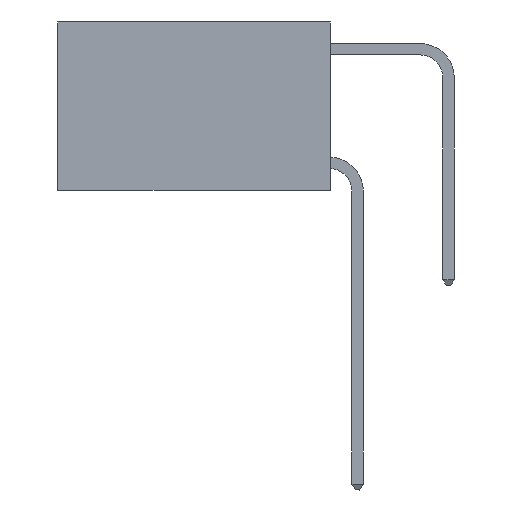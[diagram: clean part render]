
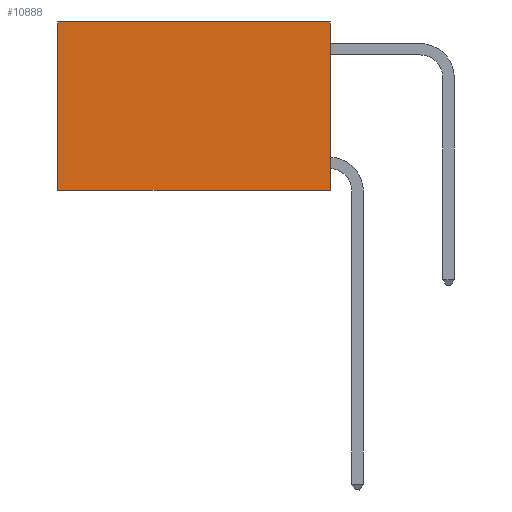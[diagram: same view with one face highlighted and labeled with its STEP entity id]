
A CAD part, left-side view. The second image highlights one B-rep face of the part: STEP entity #10888.
In plain terms, the highlighted planar face has unit normal (-1, 0, 0).
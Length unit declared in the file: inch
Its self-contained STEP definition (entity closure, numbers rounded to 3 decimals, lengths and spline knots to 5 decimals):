
#425 = DIRECTION ( 'NONE',  ( 0., 1., 0. ) ) ;
#703 = DIRECTION ( 'NONE',  ( 0., 0., -1. ) ) ;
#2368 = VECTOR ( 'NONE', #703, 39.37008 ) ;
#4046 = VERTEX_POINT ( 'NONE', #17541 ) ;
#6026 = DIRECTION ( 'NONE',  ( 1., 0., 0. ) ) ;
#7569 = VERTEX_POINT ( 'NONE', #16554 ) ;
#7814 = CARTESIAN_POINT ( 'NONE',  ( 0.2625, 0., -0.37 ) ) ;
#8562 = ORIENTED_EDGE ( 'NONE', *, *, #29483, .T. ) ;
#9877 = VECTOR ( 'NONE', #425, 39.37008 ) ;
#10718 = CARTESIAN_POINT ( 'NONE',  ( 0.2625, 0.6, 0. ) ) ;
#10888 = ADVANCED_FACE ( 'NONE', ( #12698 ), #18439, .F. ) ;
#11990 = CARTESIAN_POINT ( 'NONE',  ( 0.2625, 0., 0. ) ) ;
#12043 = VECTOR ( 'NONE', #26730, 39.37008 ) ;
#12698 = FACE_OUTER_BOUND ( 'NONE', #15386, .T. ) ;
#13679 = ORIENTED_EDGE ( 'NONE', *, *, #26137, .F. ) ;
#13909 = EDGE_CURVE ( 'NONE', #20147, #4046, #29900, .T. ) ;
#14640 = ORIENTED_EDGE ( 'NONE', *, *, #13909, .T. ) ;
#15386 = EDGE_LOOP ( 'NONE', ( #14640, #13679, #23971, #8562 ) ) ;
#16404 = EDGE_CURVE ( 'NONE', #27329, #7569, #29482, .T. ) ;
#16554 = CARTESIAN_POINT ( 'NONE',  ( 0.2625, 0., -0.37 ) ) ;
#17541 = CARTESIAN_POINT ( 'NONE',  ( 0.2625, 0.6, -0.37 ) ) ;
#18439 = PLANE ( 'NONE',  #22274 ) ;
#19445 = LINE ( 'NONE', #11990, #12043 ) ;
#20147 = VERTEX_POINT ( 'NONE', #20564 ) ;
#20564 = CARTESIAN_POINT ( 'NONE',  ( 0.2625, 0.6, 0. ) ) ;
#20909 = CARTESIAN_POINT ( 'NONE',  ( 0.2625, 0., 0. ) ) ;
#22274 = AXIS2_PLACEMENT_3D ( 'NONE', #20909, #6026, #23395 ) ;
#23068 = CARTESIAN_POINT ( 'NONE',  ( 0.2625, 0., 0. ) ) ;
#23395 = DIRECTION ( 'NONE',  ( 0., 0., -1. ) ) ;
#23871 = LINE ( 'NONE', #7814, #9877 ) ;
#23971 = ORIENTED_EDGE ( 'NONE', *, *, #16404, .F. ) ;
#24781 = CARTESIAN_POINT ( 'NONE',  ( 0.2625, 0., 0. ) ) ;
#25562 = DIRECTION ( 'NONE',  ( 0., 0., -1. ) ) ;
#26137 = EDGE_CURVE ( 'NONE', #7569, #4046, #23871, .T. ) ;
#26730 = DIRECTION ( 'NONE',  ( 0., 1., 0. ) ) ;
#27329 = VERTEX_POINT ( 'NONE', #24781 ) ;
#28383 = VECTOR ( 'NONE', #25562, 39.37008 ) ;
#29482 = LINE ( 'NONE', #23068, #2368 ) ;
#29483 = EDGE_CURVE ( 'NONE', #27329, #20147, #19445, .T. ) ;
#29900 = LINE ( 'NONE', #10718, #28383 ) ;
